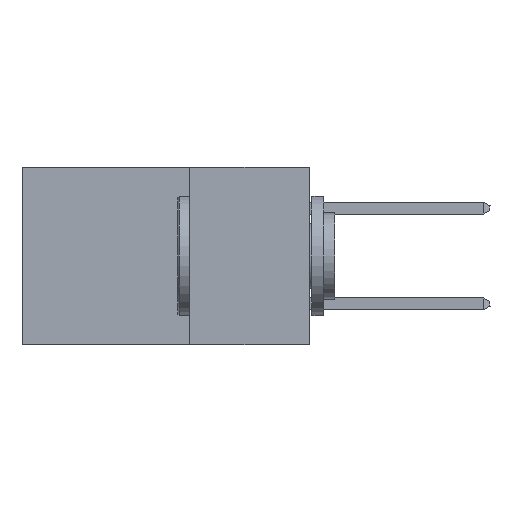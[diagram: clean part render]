
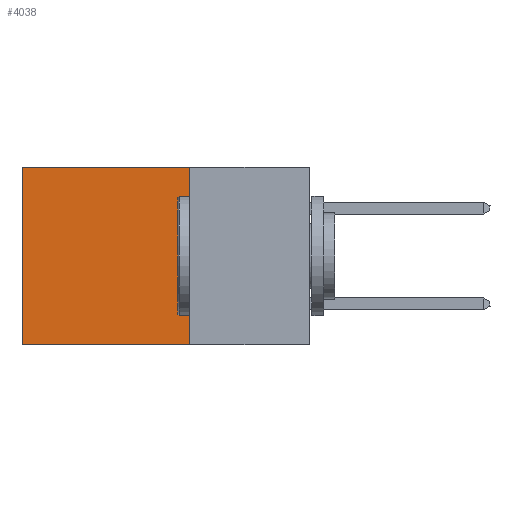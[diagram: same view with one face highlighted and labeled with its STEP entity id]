
A CAD part, left-side view. The second image highlights one B-rep face of the part: STEP entity #4038.
In plain terms, the highlighted planar face has unit normal (-1, 0, 0).
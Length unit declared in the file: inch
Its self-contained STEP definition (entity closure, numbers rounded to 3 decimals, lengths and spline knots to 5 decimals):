
#1567 = FACE_OUTER_BOUND ( 'NONE', #3279, .T. ) ;
#2093 = DIRECTION ( 'NONE',  ( 0., 1., 0. ) ) ;
#2099 = LINE ( 'NONE', #11418, #17347 ) ;
#2151 = DIRECTION ( 'NONE',  ( 0., 1., 0. ) ) ;
#2961 = VERTEX_POINT ( 'NONE', #15941 ) ;
#3070 = DIRECTION ( 'NONE',  ( 0., 0., -1. ) ) ;
#3279 = EDGE_LOOP ( 'NONE', ( #17185, #7893, #6497, #3943 ) ) ;
#3590 = EDGE_CURVE ( 'NONE', #16282, #15966, #6822, .T. ) ;
#3943 = ORIENTED_EDGE ( 'NONE', *, *, #12016, .T. ) ;
#4017 = DIRECTION ( 'NONE',  ( 0., 0., -1. ) ) ;
#4038 = ADVANCED_FACE ( 'NONE', ( #1567 ), #6875, .F. ) ;
#4747 = EDGE_CURVE ( 'NONE', #8084, #15966, #13961, .T. ) ;
#5512 = VECTOR ( 'NONE', #2093, 39.37008 ) ;
#5881 = CARTESIAN_POINT ( 'NONE',  ( 0.2875, 0.25, -0.37 ) ) ;
#6497 = ORIENTED_EDGE ( 'NONE', *, *, #7181, .F. ) ;
#6822 = LINE ( 'NONE', #16046, #9000 ) ;
#6875 = PLANE ( 'NONE',  #17854 ) ;
#7181 = EDGE_CURVE ( 'NONE', #2961, #16282, #2099, .T. ) ;
#7893 = ORIENTED_EDGE ( 'NONE', *, *, #3590, .F. ) ;
#8084 = VERTEX_POINT ( 'NONE', #10569 ) ;
#8217 = CARTESIAN_POINT ( 'NONE',  ( 0.2875, 0.25, 0. ) ) ;
#9000 = VECTOR ( 'NONE', #2151, 39.37008 ) ;
#9188 = VECTOR ( 'NONE', #4017, 39.37008 ) ;
#9809 = CARTESIAN_POINT ( 'NONE',  ( 0.2875, 0.6, 0. ) ) ;
#10569 = CARTESIAN_POINT ( 'NONE',  ( 0.2875, 0.6, 0. ) ) ;
#10981 = CARTESIAN_POINT ( 'NONE',  ( 0.2875, 0.6, -0.37 ) ) ;
#11418 = CARTESIAN_POINT ( 'NONE',  ( 0.2875, 0.25, 0. ) ) ;
#12016 = EDGE_CURVE ( 'NONE', #2961, #8084, #12659, .T. ) ;
#12501 = DIRECTION ( 'NONE',  ( 0., 0., -1. ) ) ;
#12659 = LINE ( 'NONE', #17368, #5512 ) ;
#13729 = DIRECTION ( 'NONE',  ( 1., 0., 0. ) ) ;
#13961 = LINE ( 'NONE', #9809, #9188 ) ;
#15941 = CARTESIAN_POINT ( 'NONE',  ( 0.2875, 0.25, 0. ) ) ;
#15966 = VERTEX_POINT ( 'NONE', #10981 ) ;
#16046 = CARTESIAN_POINT ( 'NONE',  ( 0.2875, 0.25, -0.37 ) ) ;
#16282 = VERTEX_POINT ( 'NONE', #5881 ) ;
#17185 = ORIENTED_EDGE ( 'NONE', *, *, #4747, .T. ) ;
#17347 = VECTOR ( 'NONE', #3070, 39.37008 ) ;
#17368 = CARTESIAN_POINT ( 'NONE',  ( 0.2875, 0.25, 0. ) ) ;
#17854 = AXIS2_PLACEMENT_3D ( 'NONE', #8217, #13729, #12501 ) ;
